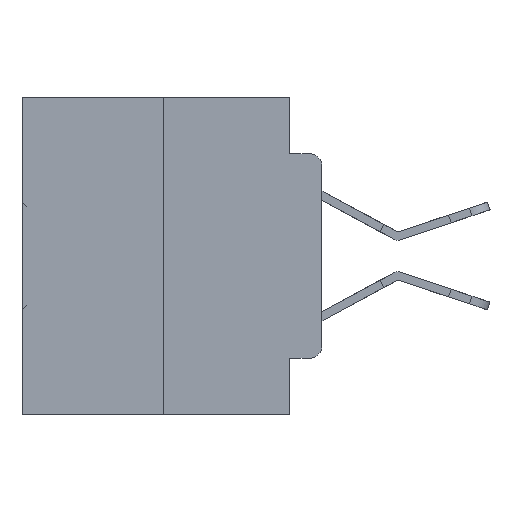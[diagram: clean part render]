
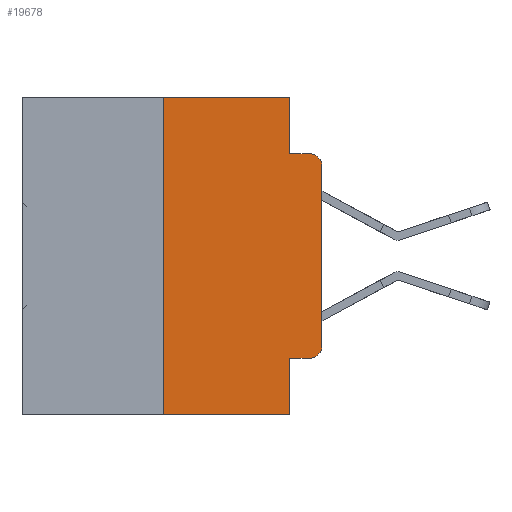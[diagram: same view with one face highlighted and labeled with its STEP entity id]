
A CAD part, left-side view. The second image highlights one B-rep face of the part: STEP entity #19678.
In plain terms, the highlighted planar face has unit normal (-1, 0, 0).
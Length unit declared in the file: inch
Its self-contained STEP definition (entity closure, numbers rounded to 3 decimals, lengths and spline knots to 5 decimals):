
#148 = ORIENTED_EDGE ( 'NONE', *, *, #12426, .F. ) ;
#306 = FACE_OUTER_BOUND ( 'NONE', #18139, .T. ) ;
#675 = CARTESIAN_POINT ( 'NONE',  ( 0., 0.25, -0.5 ) ) ;
#1582 = DIRECTION ( 'NONE',  ( 0., 0., -1. ) ) ;
#1666 = DIRECTION ( 'NONE',  ( 0., -1., 0. ) ) ;
#2117 = VECTOR ( 'NONE', #29317, 39.37008 ) ;
#2811 = CARTESIAN_POINT ( 'NONE',  ( 0., 0.051, -0.0885 ) ) ;
#2842 = VERTEX_POINT ( 'NONE', #15214 ) ;
#2979 = VERTEX_POINT ( 'NONE', #2811 ) ;
#3060 = LINE ( 'NONE', #7386, #29973 ) ;
#4096 = VERTEX_POINT ( 'NONE', #29274 ) ;
#4334 = VERTEX_POINT ( 'NONE', #28105 ) ;
#4519 = ORIENTED_EDGE ( 'NONE', *, *, #10651, .T. ) ;
#4775 = AXIS2_PLACEMENT_3D ( 'NONE', #15372, #34016, #18102 ) ;
#5018 = LINE ( 'NONE', #28667, #19434 ) ;
#6774 = VERTEX_POINT ( 'NONE', #675 ) ;
#7097 = VECTOR ( 'NONE', #31201, 39.37008 ) ;
#7386 = CARTESIAN_POINT ( 'NONE',  ( 0., 0.473, -0.5 ) ) ;
#7610 = EDGE_CURVE ( 'NONE', #4096, #2842, #26371, .T. ) ;
#7641 = CIRCLE ( 'NONE', #4775, 0.02 ) ;
#7667 = LINE ( 'NONE', #24007, #2117 ) ;
#8023 = ORIENTED_EDGE ( 'NONE', *, *, #16666, .T. ) ;
#8445 = LINE ( 'NONE', #24720, #22839 ) ;
#8632 = CARTESIAN_POINT ( 'NONE',  ( 0., 0.051, 0. ) ) ;
#8675 = PLANE ( 'NONE',  #23332 ) ;
#8827 = LINE ( 'NONE', #8632, #31043 ) ;
#9162 = ORIENTED_EDGE ( 'NONE', *, *, #34064, .F. ) ;
#9797 = CARTESIAN_POINT ( 'NONE',  ( 0., 0.25, 0. ) ) ;
#9922 = EDGE_CURVE ( 'NONE', #2842, #33159, #17948, .T. ) ;
#9958 = AXIS2_PLACEMENT_3D ( 'NONE', #33801, #17850, #1582 ) ;
#9984 = CARTESIAN_POINT ( 'NONE',  ( 0., 0.25, 0. ) ) ;
#10651 = EDGE_CURVE ( 'NONE', #6774, #19972, #3060, .T. ) ;
#12426 = EDGE_CURVE ( 'NONE', #4334, #2979, #7667, .T. ) ;
#12649 = DIRECTION ( 'NONE',  ( 0., -1., 0. ) ) ;
#14115 = DIRECTION ( 'NONE',  ( 0., 0., -1. ) ) ;
#14995 = CARTESIAN_POINT ( 'NONE',  ( 0., 0., 0. ) ) ;
#15212 = ORIENTED_EDGE ( 'NONE', *, *, #7610, .T. ) ;
#15214 = CARTESIAN_POINT ( 'NONE',  ( 0., 0., -0.3915 ) ) ;
#15222 = CARTESIAN_POINT ( 'NONE',  ( 0., 0.051, -0.4115 ) ) ;
#15372 = CARTESIAN_POINT ( 'NONE',  ( 0., 0.02, -0.1085 ) ) ;
#15462 = ORIENTED_EDGE ( 'NONE', *, *, #19662, .F. ) ;
#15862 = ORIENTED_EDGE ( 'NONE', *, *, #26813, .T. ) ;
#16666 = EDGE_CURVE ( 'NONE', #20720, #4096, #25533, .T. ) ;
#17060 = CARTESIAN_POINT ( 'NONE',  ( 0., 0.051, -0.4115 ) ) ;
#17214 = ORIENTED_EDGE ( 'NONE', *, *, #22130, .F. ) ;
#17709 = DIRECTION ( 'NONE',  ( 0., 0., 1. ) ) ;
#17850 = DIRECTION ( 'NONE',  ( -1., 0., 0. ) ) ;
#17948 = LINE ( 'NONE', #14995, #24270 ) ;
#18102 = DIRECTION ( 'NONE',  ( 0., 0., -1. ) ) ;
#18139 = EDGE_LOOP ( 'NONE', ( #21398, #15862, #15462, #148, #9162, #17214, #4519, #18559, #8023, #15212 ) ) ;
#18149 = VERTEX_POINT ( 'NONE', #9984 ) ;
#18399 = VECTOR ( 'NONE', #1666, 39.37008 ) ;
#18559 = ORIENTED_EDGE ( 'NONE', *, *, #20334, .F. ) ;
#19434 = VECTOR ( 'NONE', #12649, 39.37008 ) ;
#19662 = EDGE_CURVE ( 'NONE', #2979, #34292, #8445, .T. ) ;
#19678 = ADVANCED_FACE ( 'NONE', ( #306 ), #8675, .F. ) ;
#19972 = VERTEX_POINT ( 'NONE', #25858 ) ;
#20334 = EDGE_CURVE ( 'NONE', #20720, #19972, #8827, .T. ) ;
#20720 = VERTEX_POINT ( 'NONE', #17060 ) ;
#21398 = ORIENTED_EDGE ( 'NONE', *, *, #9922, .T. ) ;
#21512 = LINE ( 'NONE', #9797, #7097 ) ;
#22130 = EDGE_CURVE ( 'NONE', #6774, #18149, #21512, .T. ) ;
#22376 = CARTESIAN_POINT ( 'NONE',  ( 0., 0., -0.1085 ) ) ;
#22839 = VECTOR ( 'NONE', #30007, 39.37008 ) ;
#23332 = AXIS2_PLACEMENT_3D ( 'NONE', #27499, #30122, #14115 ) ;
#23576 = DIRECTION ( 'NONE',  ( 0., -1., 0. ) ) ;
#24007 = CARTESIAN_POINT ( 'NONE',  ( 0., 0.051, 0. ) ) ;
#24270 = VECTOR ( 'NONE', #17709, 39.37008 ) ;
#24720 = CARTESIAN_POINT ( 'NONE',  ( 0., 0.051, -0.0885 ) ) ;
#25533 = LINE ( 'NONE', #15222, #18399 ) ;
#25858 = CARTESIAN_POINT ( 'NONE',  ( 0., 0.051, -0.5 ) ) ;
#26371 = CIRCLE ( 'NONE', #9958, 0.02 ) ;
#26813 = EDGE_CURVE ( 'NONE', #33159, #34292, #7641, .T. ) ;
#27456 = DIRECTION ( 'NONE',  ( 0., 0., -1. ) ) ;
#27499 = CARTESIAN_POINT ( 'NONE',  ( 0., 0.473, 0. ) ) ;
#28105 = CARTESIAN_POINT ( 'NONE',  ( 0., 0.051, 0. ) ) ;
#28667 = CARTESIAN_POINT ( 'NONE',  ( 0., 0.473, 0. ) ) ;
#29274 = CARTESIAN_POINT ( 'NONE',  ( 0., 0.02, -0.4115 ) ) ;
#29317 = DIRECTION ( 'NONE',  ( 0., 0., -1. ) ) ;
#29561 = CARTESIAN_POINT ( 'NONE',  ( 0., 0.02, -0.0885 ) ) ;
#29973 = VECTOR ( 'NONE', #23576, 39.37008 ) ;
#30007 = DIRECTION ( 'NONE',  ( 0., -1., 0. ) ) ;
#30122 = DIRECTION ( 'NONE',  ( 1., 0., 0. ) ) ;
#31043 = VECTOR ( 'NONE', #27456, 39.37008 ) ;
#31201 = DIRECTION ( 'NONE',  ( 0., 0., 1. ) ) ;
#33159 = VERTEX_POINT ( 'NONE', #22376 ) ;
#33801 = CARTESIAN_POINT ( 'NONE',  ( 0., 0.02, -0.3915 ) ) ;
#34016 = DIRECTION ( 'NONE',  ( -1., 0., 0. ) ) ;
#34064 = EDGE_CURVE ( 'NONE', #18149, #4334, #5018, .T. ) ;
#34292 = VERTEX_POINT ( 'NONE', #29561 ) ;
